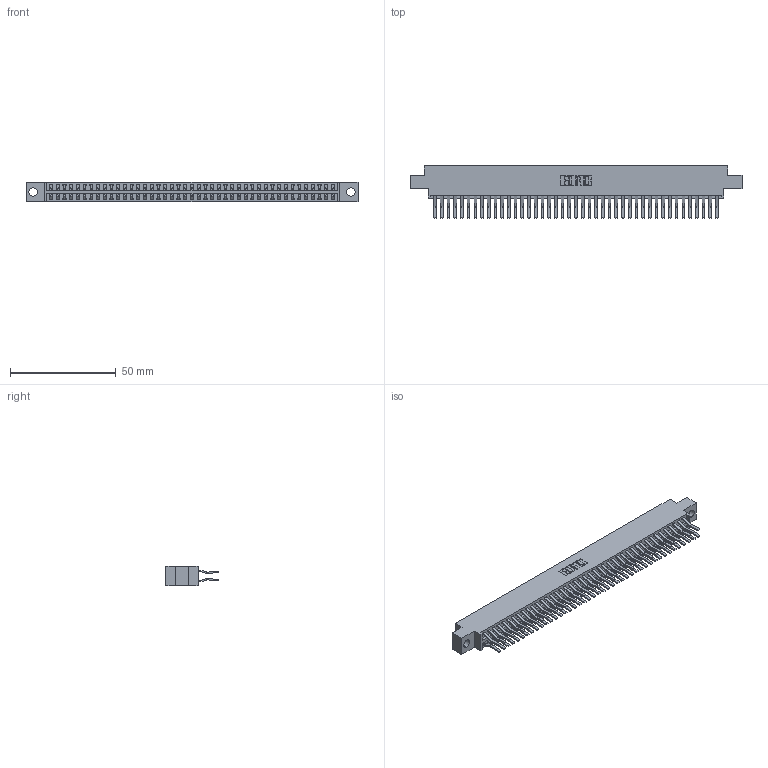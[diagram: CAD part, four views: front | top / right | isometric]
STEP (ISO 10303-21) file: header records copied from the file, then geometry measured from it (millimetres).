
FILE_DESCRIPTION (( 'STEP AP203' ), '1' );
FILE_NAME ('346-086-560-804.STEP', '2022-05-25T23:52:27', ( '' ), ( '' ), 'SwSTEP 2.0', 'SolidWorks 2020', '' );
FILE_SCHEMA (( 'CONFIG_CONTROL_DESIGN' ));
Length unit declared in the file: inch
Products named in the file (3): 345-292-001_560 Tail; 346-086-560-804; 346 Part_0.170 Offset - 0.156 Dia-TH
Assembly tree (87 placements, depth 2):
  346-086-560-804
    346 Part_0.170 Offset - 0.156 Dia-TH
    345-292-001_560 Tail  x86
Bounding box: 157.1 x 24.78 x 9.4 mm (x, y, z)
Volume: 15630 mm3; surface area: 23031.6 mm2
Topology: 87 solids, 87 shells, 4784 faces, 14223 edges, 9366 vertices
Faces by surface type: plane 3104, cylinder 1680
Entity records: 28567 total; most frequent: CARTESIAN_POINT 4714, ORIENTED_EDGE 4646, DIRECTION 4207, EDGE_CURVE 2323, VECTOR 2015, LINE 2015, VERTEX_POINT 1546, AXIS2_PLACEMENT_3D 1096
